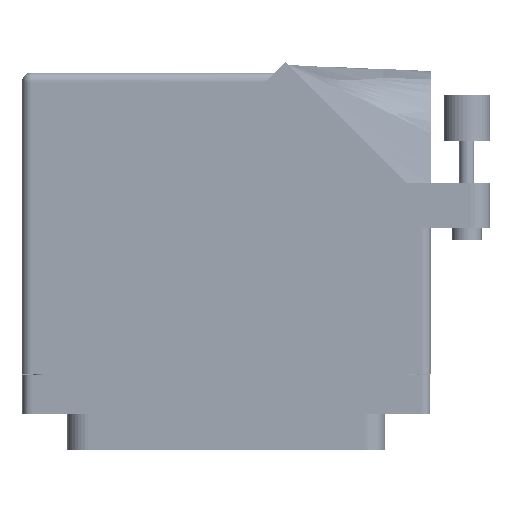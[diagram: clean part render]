
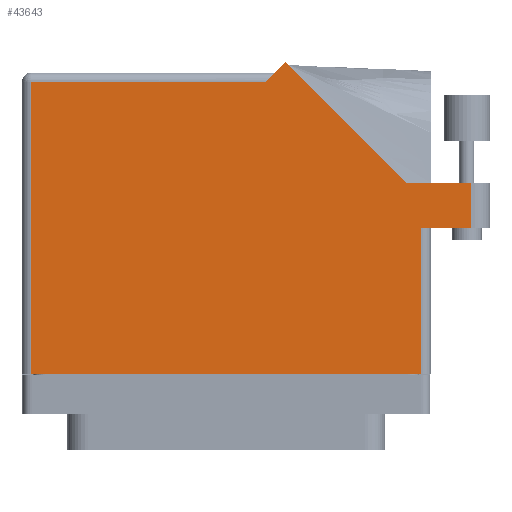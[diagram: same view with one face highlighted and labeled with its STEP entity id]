
A CAD part, front view. The second image highlights one B-rep face of the part: STEP entity #43643.
In plain terms, the highlighted face is planar.
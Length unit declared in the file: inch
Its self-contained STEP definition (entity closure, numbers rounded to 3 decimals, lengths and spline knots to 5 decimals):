
#1274 = ORIENTED_EDGE ( 'NONE', *, *, #24492, .T. ) ;
#1288 = ORIENTED_EDGE ( 'NONE', *, *, #33703, .T. ) ;
#1466 = EDGE_LOOP ( 'NONE', ( #91271, #71303, #1288, #28196, #13458, #1274, #34810, #35250, #34573 ) ) ;
#2029 = VECTOR ( 'NONE', #41631, 39.37008 ) ;
#3603 = EDGE_CURVE ( 'NONE', #9306, #64324, #45173, .T. ) ;
#4494 = CARTESIAN_POINT ( 'NONE',  ( -1.3155, -0.1, 0.765 ) ) ;
#5403 = DIRECTION ( 'NONE',  ( -1., 0., 0. ) ) ;
#6410 = CARTESIAN_POINT ( 'NONE',  ( 1.3775, 0.88, 0.765 ) ) ;
#6579 = LINE ( 'NONE', #6410, #2029 ) ;
#6871 = EDGE_CURVE ( 'NONE', #20081, #52791, #69661, .T. ) ;
#7190 = LINE ( 'NONE', #72868, #92538 ) ;
#9306 = VERTEX_POINT ( 'NONE', #26130 ) ;
#10153 = CARTESIAN_POINT ( 'NONE',  ( 0.2655, 1.868, 0.765 ) ) ;
#13169 = CARTESIAN_POINT ( 'NONE',  ( -1.3775, -0.1, 0.765 ) ) ;
#13458 = ORIENTED_EDGE ( 'NONE', *, *, #41500, .T. ) ;
#19059 = CARTESIAN_POINT ( 'NONE',  ( 0.39821, 2.00071, 0.765 ) ) ;
#20081 = VERTEX_POINT ( 'NONE', #56441 ) ;
#20644 = DIRECTION ( 'NONE',  ( -1., 0., 0. ) ) ;
#20898 = LINE ( 'NONE', #84362, #32168 ) ;
#24492 = EDGE_CURVE ( 'NONE', #40157, #49025, #7190, .T. ) ;
#26130 = CARTESIAN_POINT ( 'NONE',  ( 1.21192, 1.187, 0.765 ) ) ;
#26183 = EDGE_CURVE ( 'NONE', #52791, #29146, #6579, .T. ) ;
#27020 = CARTESIAN_POINT ( 'NONE',  ( 1.3155, 0.88, 0.765 ) ) ;
#28096 = DIRECTION ( 'NONE',  ( -0.707, -0.707, 0. ) ) ;
#28196 = ORIENTED_EDGE ( 'NONE', *, *, #3603, .T. ) ;
#28487 = VECTOR ( 'NONE', #77071, 39.37008 ) ;
#29146 = VERTEX_POINT ( 'NONE', #38471 ) ;
#29481 = EDGE_CURVE ( 'NONE', #29146, #40543, #41957, .T. ) ;
#32168 = VECTOR ( 'NONE', #20644, 39.37008 ) ;
#33406 = DIRECTION ( 'NONE',  ( 0., -1., 0. ) ) ;
#33703 = EDGE_CURVE ( 'NONE', #40543, #9306, #20898, .T. ) ;
#34573 = ORIENTED_EDGE ( 'NONE', *, *, #6871, .T. ) ;
#34810 = ORIENTED_EDGE ( 'NONE', *, *, #41705, .T. ) ;
#35250 = ORIENTED_EDGE ( 'NONE', *, *, #36753, .T. ) ;
#36753 = EDGE_CURVE ( 'NONE', #81728, #20081, #71097, .T. ) ;
#37010 = DIRECTION ( 'NONE',  ( -1., 0., 0. ) ) ;
#37285 = CARTESIAN_POINT ( 'NONE',  ( 1.21192, 1.187, 0.765 ) ) ;
#38471 = CARTESIAN_POINT ( 'NONE',  ( 1.6525, 0.88, 0.765 ) ) ;
#40157 = VERTEX_POINT ( 'NONE', #10153 ) ;
#40543 = VERTEX_POINT ( 'NONE', #69509 ) ;
#41500 = EDGE_CURVE ( 'NONE', #64324, #40157, #84436, .T. ) ;
#41546 = DIRECTION ( 'NONE',  ( 0., 0., -1. ) ) ;
#41631 = DIRECTION ( 'NONE',  ( 1., 0., 0. ) ) ;
#41705 = EDGE_CURVE ( 'NONE', #49025, #81728, #45080, .T. ) ;
#41957 = LINE ( 'NONE', #55367, #28487 ) ;
#42006 = DIRECTION ( 'NONE',  ( -0.707, 0.707, 0. ) ) ;
#43643 = ADVANCED_FACE ( 'NONE', ( #64907 ), #49045, .F. ) ;
#45080 = LINE ( 'NONE', #4494, #70997 ) ;
#45173 = LINE ( 'NONE', #37285, #90087 ) ;
#47906 = CARTESIAN_POINT ( 'NONE',  ( 1.3155, 0.88, 0.765 ) ) ;
#49025 = VERTEX_POINT ( 'NONE', #71296 ) ;
#49045 = PLANE ( 'NONE',  #71230 ) ;
#52791 = VERTEX_POINT ( 'NONE', #47906 ) ;
#55367 = CARTESIAN_POINT ( 'NONE',  ( 1.6525, 1.187, 0.765 ) ) ;
#56441 = CARTESIAN_POINT ( 'NONE',  ( 1.3155, -0.1, 0.765 ) ) ;
#62012 = VECTOR ( 'NONE', #84737, 39.37008 ) ;
#62516 = DIRECTION ( 'NONE',  ( 0., 1., 0. ) ) ;
#64324 = VERTEX_POINT ( 'NONE', #19059 ) ;
#64907 = FACE_OUTER_BOUND ( 'NONE', #1466, .T. ) ;
#69509 = CARTESIAN_POINT ( 'NONE',  ( 1.6525, 1.187, 0.765 ) ) ;
#69661 = LINE ( 'NONE', #27020, #71942 ) ;
#70580 = CARTESIAN_POINT ( 'NONE',  ( 0.3275, 1.93, 0.765 ) ) ;
#70997 = VECTOR ( 'NONE', #33406, 39.37008 ) ;
#71097 = LINE ( 'NONE', #13169, #62012 ) ;
#71230 = AXIS2_PLACEMENT_3D ( 'NONE', #92319, #41546, #5403 ) ;
#71296 = CARTESIAN_POINT ( 'NONE',  ( -1.3155, 1.868, 0.765 ) ) ;
#71303 = ORIENTED_EDGE ( 'NONE', *, *, #29481, .T. ) ;
#71942 = VECTOR ( 'NONE', #62516, 39.37008 ) ;
#72868 = CARTESIAN_POINT ( 'NONE',  ( -1.3775, 1.868, 0.765 ) ) ;
#73238 = VECTOR ( 'NONE', #28096, 39.37008 ) ;
#77071 = DIRECTION ( 'NONE',  ( 0., 1., 0. ) ) ;
#81728 = VERTEX_POINT ( 'NONE', #91520 ) ;
#84362 = CARTESIAN_POINT ( 'NONE',  ( 1.7775, 1.187, 0.765 ) ) ;
#84436 = LINE ( 'NONE', #70580, #73238 ) ;
#84737 = DIRECTION ( 'NONE',  ( 1., 0., 0. ) ) ;
#90087 = VECTOR ( 'NONE', #42006, 39.37008 ) ;
#91271 = ORIENTED_EDGE ( 'NONE', *, *, #26183, .T. ) ;
#91520 = CARTESIAN_POINT ( 'NONE',  ( -1.3155, -0.1, 0.765 ) ) ;
#92319 = CARTESIAN_POINT ( 'NONE',  ( -1.3775, 1.93, 0.765 ) ) ;
#92538 = VECTOR ( 'NONE', #37010, 39.37008 ) ;
